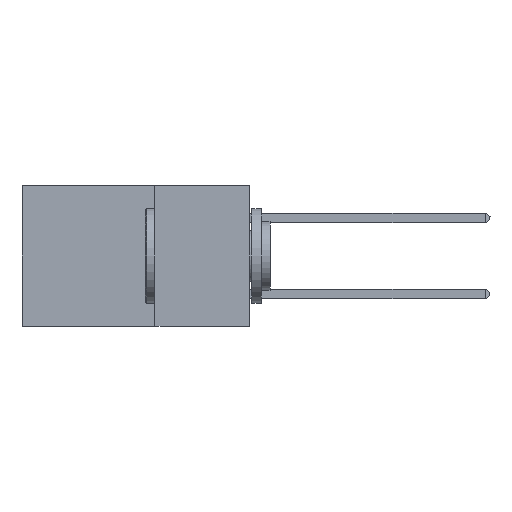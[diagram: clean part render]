
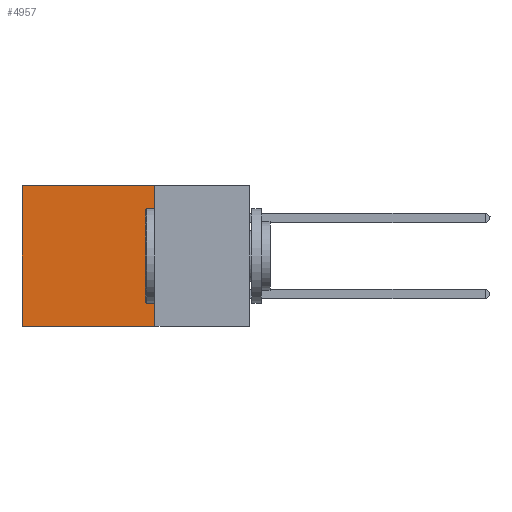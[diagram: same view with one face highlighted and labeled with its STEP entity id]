
A CAD part, left-side view. The second image highlights one B-rep face of the part: STEP entity #4957.
In plain terms, the highlighted planar face has unit normal (-1, 0, 0).
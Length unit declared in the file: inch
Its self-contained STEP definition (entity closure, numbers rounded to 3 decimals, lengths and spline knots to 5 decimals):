
#60 = ORIENTED_EDGE ( 'NONE', *, *, #18805, .T. ) ;
#590 = CARTESIAN_POINT ( 'NONE',  ( 0.2875, 0.25, 0. ) ) ;
#2264 = VERTEX_POINT ( 'NONE', #3124 ) ;
#2773 = EDGE_CURVE ( 'NONE', #15970, #2264, #15323, .T. ) ;
#3124 = CARTESIAN_POINT ( 'NONE',  ( 0.2875, 0.25, -0.37 ) ) ;
#3381 = VERTEX_POINT ( 'NONE', #4435 ) ;
#4435 = CARTESIAN_POINT ( 'NONE',  ( 0.2875, 0.6, -0.37 ) ) ;
#4957 = ADVANCED_FACE ( 'NONE', ( #10920 ), #18859, .F. ) ;
#5148 = ORIENTED_EDGE ( 'NONE', *, *, #15309, .F. ) ;
#7163 = CARTESIAN_POINT ( 'NONE',  ( 0.2875, 0.25, 0. ) ) ;
#7176 = VECTOR ( 'NONE', #22969, 39.37008 ) ;
#7995 = DIRECTION ( 'NONE',  ( 0., 0., -1. ) ) ;
#8213 = LINE ( 'NONE', #17762, #14638 ) ;
#9096 = DIRECTION ( 'NONE',  ( 1., 0., 0. ) ) ;
#9486 = VECTOR ( 'NONE', #21981, 39.37008 ) ;
#10920 = FACE_OUTER_BOUND ( 'NONE', #22422, .T. ) ;
#11041 = AXIS2_PLACEMENT_3D ( 'NONE', #7163, #9096, #22716 ) ;
#11123 = CARTESIAN_POINT ( 'NONE',  ( 0.2875, 0.25, 0. ) ) ;
#12208 = DIRECTION ( 'NONE',  ( 0., 1., 0. ) ) ;
#12359 = LINE ( 'NONE', #22886, #7176 ) ;
#14109 = ORIENTED_EDGE ( 'NONE', *, *, #17050, .T. ) ;
#14638 = VECTOR ( 'NONE', #7995, 39.37008 ) ;
#15286 = CARTESIAN_POINT ( 'NONE',  ( 0.2875, 0.6, 0. ) ) ;
#15309 = EDGE_CURVE ( 'NONE', #2264, #3381, #12359, .T. ) ;
#15318 = VERTEX_POINT ( 'NONE', #15286 ) ;
#15323 = LINE ( 'NONE', #20053, #9486 ) ;
#15970 = VERTEX_POINT ( 'NONE', #11123 ) ;
#16334 = ORIENTED_EDGE ( 'NONE', *, *, #2773, .F. ) ;
#17050 = EDGE_CURVE ( 'NONE', #15970, #15318, #18103, .T. ) ;
#17762 = CARTESIAN_POINT ( 'NONE',  ( 0.2875, 0.6, 0. ) ) ;
#18103 = LINE ( 'NONE', #590, #22597 ) ;
#18805 = EDGE_CURVE ( 'NONE', #15318, #3381, #8213, .T. ) ;
#18859 = PLANE ( 'NONE',  #11041 ) ;
#20053 = CARTESIAN_POINT ( 'NONE',  ( 0.2875, 0.25, 0. ) ) ;
#21981 = DIRECTION ( 'NONE',  ( 0., 0., -1. ) ) ;
#22422 = EDGE_LOOP ( 'NONE', ( #60, #5148, #16334, #14109 ) ) ;
#22597 = VECTOR ( 'NONE', #12208, 39.37008 ) ;
#22716 = DIRECTION ( 'NONE',  ( 0., 0., -1. ) ) ;
#22886 = CARTESIAN_POINT ( 'NONE',  ( 0.2875, 0.25, -0.37 ) ) ;
#22969 = DIRECTION ( 'NONE',  ( 0., 1., 0. ) ) ;
